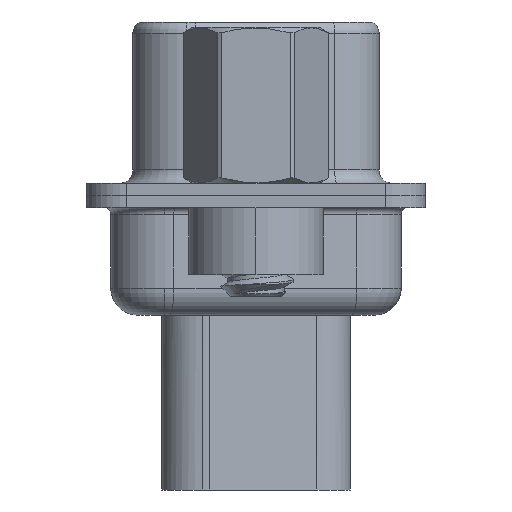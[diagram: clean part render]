
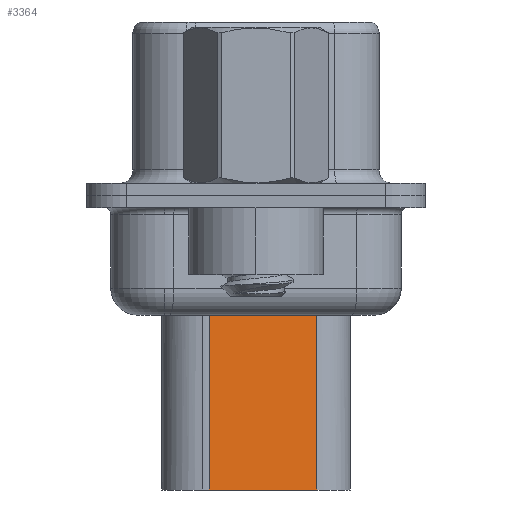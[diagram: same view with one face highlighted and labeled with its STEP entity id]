
A CAD part, left-side view. The second image highlights one B-rep face of the part: STEP entity #3364.
In plain terms, the highlighted planar face has unit normal (-0.985, -0.174, 0).
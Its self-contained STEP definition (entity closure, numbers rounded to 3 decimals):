
#561 = FACE_OUTER_BOUND ( 'NONE', #17651, .T. ) ;
#866 = CARTESIAN_POINT ( 'NONE',  ( 4.524, 1.74, -3.1 ) ) ;
#1032 = VECTOR ( 'NONE', #3028, 1000. ) ;
#2186 = ORIENTED_EDGE ( 'NONE', *, *, #22370, .T. ) ;
#2392 = EDGE_CURVE ( 'NONE', #12721, #4612, #14982, .T. ) ;
#3028 = DIRECTION ( 'NONE',  ( -0.174, 0.985, 0. ) ) ;
#3364 = ADVANCED_FACE ( 'NONE', ( #561 ), #20170, .T. ) ;
#4612 = VERTEX_POINT ( 'NONE', #17750 ) ;
#5427 = VECTOR ( 'NONE', #13889, 1000. ) ;
#6012 = DIRECTION ( 'NONE',  ( -0.985, -0.174, 0. ) ) ;
#6286 = VECTOR ( 'NONE', #18485, 1000. ) ;
#6792 = AXIS2_PLACEMENT_3D ( 'NONE', #9725, #6012, #7650 ) ;
#6838 = CARTESIAN_POINT ( 'NONE',  ( 5.229, -2.26, -3.1 ) ) ;
#7650 = DIRECTION ( 'NONE',  ( 0.174, -0.985, 0. ) ) ;
#8562 = LINE ( 'NONE', #6838, #5427 ) ;
#9725 = CARTESIAN_POINT ( 'NONE',  ( 4.524, 1.74, -3.1 ) ) ;
#11280 = CARTESIAN_POINT ( 'NONE',  ( 4.524, 1.74, -10.95 ) ) ;
#11437 = LINE ( 'NONE', #866, #19338 ) ;
#12721 = VERTEX_POINT ( 'NONE', #16257 ) ;
#13641 = ORIENTED_EDGE ( 'NONE', *, *, #14642, .T. ) ;
#13889 = DIRECTION ( 'NONE',  ( 0., 0., -1. ) ) ;
#14642 = EDGE_CURVE ( 'NONE', #18975, #4612, #11437, .T. ) ;
#14982 = LINE ( 'NONE', #11280, #6286 ) ;
#15333 = LINE ( 'NONE', #15558, #1032 ) ;
#15558 = CARTESIAN_POINT ( 'NONE',  ( 4.353, 2.709, -3.975 ) ) ;
#16257 = CARTESIAN_POINT ( 'NONE',  ( 5.229, -2.26, -10.95 ) ) ;
#17625 = ORIENTED_EDGE ( 'NONE', *, *, #20016, .F. ) ;
#17651 = EDGE_LOOP ( 'NONE', ( #17625, #2186, #13641, #21958 ) ) ;
#17750 = CARTESIAN_POINT ( 'NONE',  ( 4.524, 1.74, -10.95 ) ) ;
#18342 = VERTEX_POINT ( 'NONE', #22164 ) ;
#18453 = CARTESIAN_POINT ( 'NONE',  ( 4.524, 1.74, -3.975 ) ) ;
#18485 = DIRECTION ( 'NONE',  ( -0.174, 0.985, 0. ) ) ;
#18975 = VERTEX_POINT ( 'NONE', #18453 ) ;
#19338 = VECTOR ( 'NONE', #20143, 1000. ) ;
#20016 = EDGE_CURVE ( 'NONE', #18342, #12721, #8562, .T. ) ;
#20143 = DIRECTION ( 'NONE',  ( 0., 0., -1. ) ) ;
#20170 = PLANE ( 'NONE',  #6792 ) ;
#21958 = ORIENTED_EDGE ( 'NONE', *, *, #2392, .F. ) ;
#22164 = CARTESIAN_POINT ( 'NONE',  ( 5.229, -2.26, -3.975 ) ) ;
#22370 = EDGE_CURVE ( 'NONE', #18342, #18975, #15333, .T. ) ;
